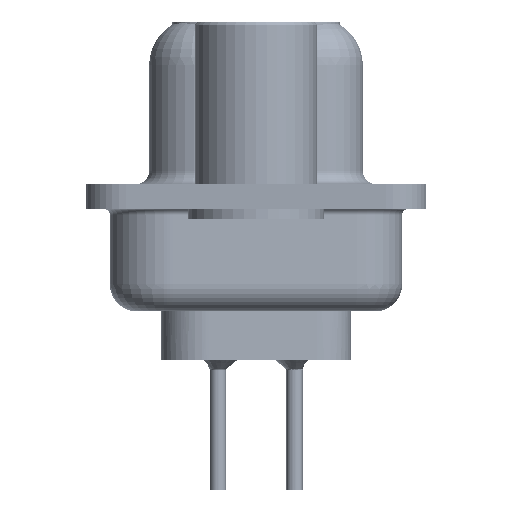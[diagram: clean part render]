
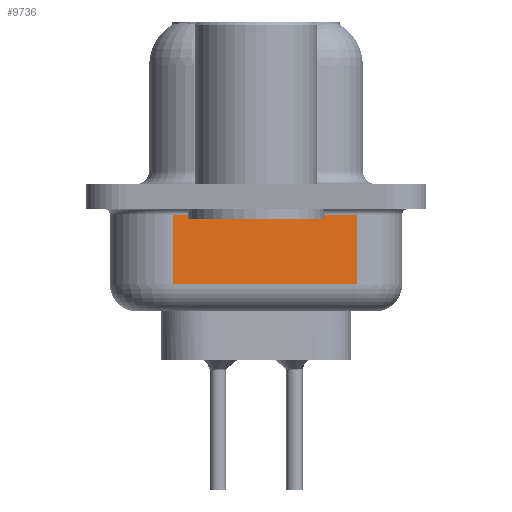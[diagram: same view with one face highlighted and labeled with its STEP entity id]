
A CAD part, left-side view. The second image highlights one B-rep face of the part: STEP entity #9736.
In plain terms, the highlighted planar face has unit normal (-0.985, -0.174, 0).
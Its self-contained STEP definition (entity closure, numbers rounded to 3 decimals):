
#2221 = CARTESIAN_POINT ( 'NONE',  ( 4.079, -3.747, -0.7 ) ) ;
#3836 = DIRECTION ( 'NONE',  ( 0.985, 0.174, 0. ) ) ;
#5898 = EDGE_CURVE ( 'NONE', #32968, #14777, #19475, .T. ) ;
#5913 = CARTESIAN_POINT ( 'NONE',  ( 2.88, 3.053, -4.25 ) ) ;
#6242 = DIRECTION ( 'NONE',  ( 0.174, -0.985, 0. ) ) ;
#6620 = ORIENTED_EDGE ( 'NONE', *, *, #18597, .F. ) ;
#6733 = LINE ( 'NONE', #9115, #28590 ) ;
#7863 = ORIENTED_EDGE ( 'NONE', *, *, #18714, .T. ) ;
#8164 = CARTESIAN_POINT ( 'NONE',  ( 4.079, -3.747, -3.25 ) ) ;
#8434 = CARTESIAN_POINT ( 'NONE',  ( 2.88, 3.053, -3.25 ) ) ;
#8446 = PLANE ( 'NONE',  #16398 ) ;
#9115 = CARTESIAN_POINT ( 'NONE',  ( 4.079, -3.747, -4.25 ) ) ;
#9736 = ADVANCED_FACE ( 'NONE', ( #27146 ), #8446, .F. ) ;
#10734 = VERTEX_POINT ( 'NONE', #13230 ) ;
#10905 = ORIENTED_EDGE ( 'NONE', *, *, #20973, .T. ) ;
#12807 = LINE ( 'NONE', #15344, #33051 ) ;
#13230 = CARTESIAN_POINT ( 'NONE',  ( 2.88, 3.053, -0.7 ) ) ;
#13437 = CARTESIAN_POINT ( 'NONE',  ( 2.88, 3.053, -4.25 ) ) ;
#14777 = VERTEX_POINT ( 'NONE', #8164 ) ;
#15344 = CARTESIAN_POINT ( 'NONE',  ( 2.88, 3.053, -0.7 ) ) ;
#16398 = AXIS2_PLACEMENT_3D ( 'NONE', #5913, #3836, #24601 ) ;
#16926 = CARTESIAN_POINT ( 'NONE',  ( 2.88, 3.053, -3.25 ) ) ;
#17084 = DIRECTION ( 'NONE',  ( 0., 0., 1. ) ) ;
#18597 = EDGE_CURVE ( 'NONE', #32968, #10734, #20895, .T. ) ;
#18714 = EDGE_CURVE ( 'NONE', #14777, #25449, #6733, .T. ) ;
#19475 = LINE ( 'NONE', #8434, #24136 ) ;
#20895 = LINE ( 'NONE', #13437, #29097 ) ;
#20973 = EDGE_CURVE ( 'NONE', #25449, #10734, #12807, .T. ) ;
#22349 = EDGE_LOOP ( 'NONE', ( #6620, #29834, #7863, #10905 ) ) ;
#24136 = VECTOR ( 'NONE', #6242, 1000. ) ;
#24601 = DIRECTION ( 'NONE',  ( -0.174, 0.985, 0. ) ) ;
#25449 = VERTEX_POINT ( 'NONE', #2221 ) ;
#26031 = DIRECTION ( 'NONE',  ( 0., 0., 1. ) ) ;
#27146 = FACE_OUTER_BOUND ( 'NONE', #22349, .T. ) ;
#28590 = VECTOR ( 'NONE', #17084, 1000. ) ;
#29097 = VECTOR ( 'NONE', #26031, 1000. ) ;
#29834 = ORIENTED_EDGE ( 'NONE', *, *, #5898, .T. ) ;
#32968 = VERTEX_POINT ( 'NONE', #16926 ) ;
#33051 = VECTOR ( 'NONE', #33397, 1000. ) ;
#33397 = DIRECTION ( 'NONE',  ( -0.174, 0.985, 0. ) ) ;
